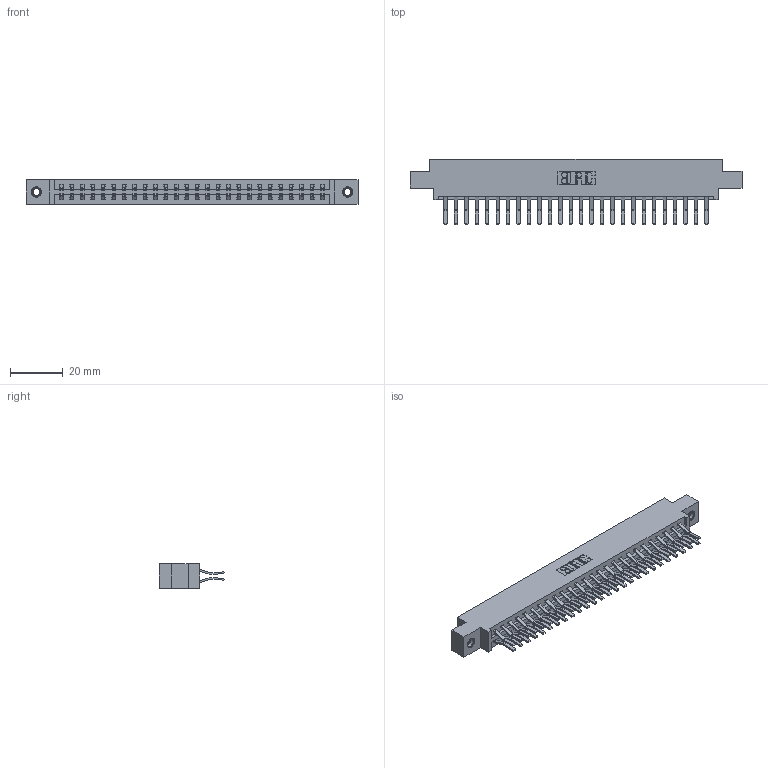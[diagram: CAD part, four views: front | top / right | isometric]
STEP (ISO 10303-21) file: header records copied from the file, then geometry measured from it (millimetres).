
FILE_DESCRIPTION (( 'STEP AP203' ), '1' );
FILE_NAME ('387-052-560-807.STEP', '2019-10-19T04:14:56', ( '' ), ( '' ), 'SwSTEP 2.0', 'SolidWorks 2016', '' );
FILE_SCHEMA (( 'CONFIG_CONTROL_DESIGN' ));
Length unit declared in the file: inch
Products named in the file (4): 337 Part_0.170 Offset - 0.156 Dia-TI; 345-250-001_345-250-005-103; 345-292-001_560 Tail; 387-052-560-807
Assembly tree (55 placements, depth 2):
  387-052-560-807
    337 Part_0.170 Offset - 0.156 Dia-TI
    345-292-001_560 Tail  x52
    345-250-001_345-250-005-103  x2
Bounding box: 126.03 x 24.78 x 9.4 mm (x, y, z)
Volume: 13279.4 mm3; surface area: 15987.2 mm2
Topology: 55 solids, 55 shells, 3090 faces, 9143 edges, 6018 vertices
Faces by surface type: plane 2082, cylinder 992, cone 12, torus 4
Entity records: 23634 total; most frequent: CARTESIAN_POINT 3977, ORIENTED_EDGE 3906, DIRECTION 3447, EDGE_CURVE 1953, LINE 1801, VECTOR 1801, VERTEX_POINT 1296, AXIS2_PLACEMENT_3D 823
